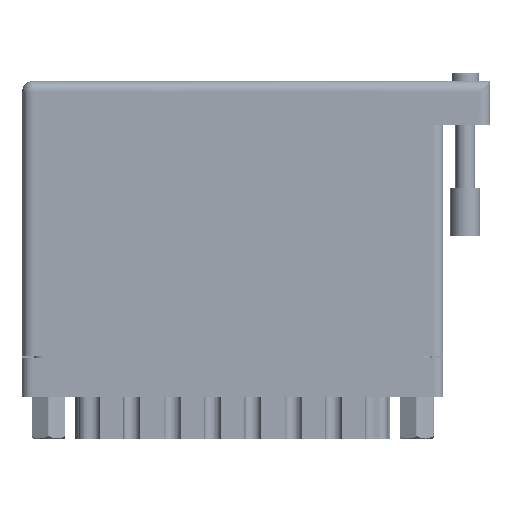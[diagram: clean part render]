
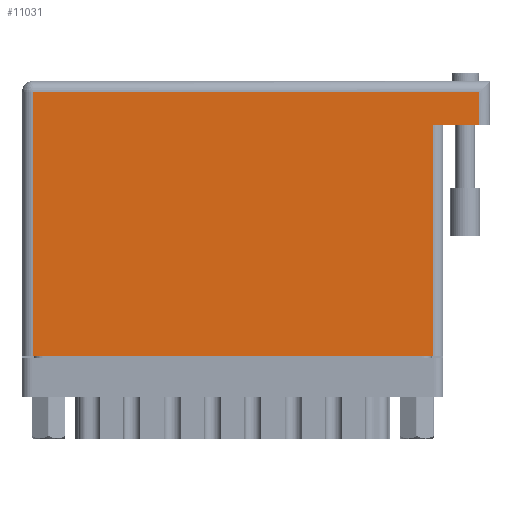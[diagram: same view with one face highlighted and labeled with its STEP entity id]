
A CAD part, front view. The second image highlights one B-rep face of the part: STEP entity #11031.
In plain terms, the highlighted face is planar.
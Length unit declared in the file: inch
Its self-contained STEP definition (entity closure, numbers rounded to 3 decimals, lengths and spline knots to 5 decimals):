
#3420 = ORIENTED_EDGE ( 'NONE', *, *, #61416, .T. ) ;
#5958 = DIRECTION ( 'NONE',  ( 1., 0., 0. ) ) ;
#5983 = AXIS2_PLACEMENT_3D ( 'NONE', #17333, #24297, #83875 ) ;
#5984 = EDGE_CURVE ( 'NONE', #15269, #26244, #51164, .T. ) ;
#6427 = CARTESIAN_POINT ( 'NONE',  ( 0.07, 0., 0. ) ) ;
#7110 = DIRECTION ( 'NONE',  ( 0., 1., 0. ) ) ;
#8428 = ORIENTED_EDGE ( 'NONE', *, *, #5984, .T. ) ;
#8669 = FACE_OUTER_BOUND ( 'NONE', #66862, .T. ) ;
#9192 = LINE ( 'NONE', #63873, #42277 ) ;
#9194 = LINE ( 'NONE', #27393, #59892 ) ;
#9333 = EDGE_CURVE ( 'NONE', #26244, #36953, #9194, .T. ) ;
#11031 = ADVANCED_FACE ( 'NONE', ( #8669 ), #83304, .F. ) ;
#11588 = VERTEX_POINT ( 'NONE', #49985 ) ;
#12698 = LINE ( 'NONE', #33693, #57027 ) ;
#13723 = DIRECTION ( 'NONE',  ( -1., 0., 0. ) ) ;
#15269 = VERTEX_POINT ( 'NONE', #6427 ) ;
#17333 = CARTESIAN_POINT ( 'NONE',  ( 0., 1.775, 0. ) ) ;
#22354 = ORIENTED_EDGE ( 'NONE', *, *, #35326, .T. ) ;
#23935 = EDGE_CURVE ( 'NONE', #74071, #11588, #73163, .T. ) ;
#24273 = DIRECTION ( 'NONE',  ( 0., -1., 0. ) ) ;
#24297 = DIRECTION ( 'NONE',  ( 0., 0., -1. ) ) ;
#25560 = EDGE_CURVE ( 'NONE', #74071, #36953, #12698, .T. ) ;
#26244 = VERTEX_POINT ( 'NONE', #29284 ) ;
#27393 = CARTESIAN_POINT ( 'NONE',  ( 2.648, 1.495, 0. ) ) ;
#29284 = CARTESIAN_POINT ( 'NONE',  ( 2.648, 0., 0. ) ) ;
#32236 = ORIENTED_EDGE ( 'NONE', *, *, #25560, .F. ) ;
#33693 = CARTESIAN_POINT ( 'NONE',  ( 3.018, 1.495, 0. ) ) ;
#35326 = EDGE_CURVE ( 'NONE', #11588, #36630, #79288, .T. ) ;
#36630 = VERTEX_POINT ( 'NONE', #47289 ) ;
#36953 = VERTEX_POINT ( 'NONE', #84575 ) ;
#42277 = VECTOR ( 'NONE', #24273, 39.37008 ) ;
#47289 = CARTESIAN_POINT ( 'NONE',  ( 0.07, 1.705, 0. ) ) ;
#49985 = CARTESIAN_POINT ( 'NONE',  ( 2.948, 1.705, 0. ) ) ;
#51164 = LINE ( 'NONE', #84972, #66567 ) ;
#52670 = ORIENTED_EDGE ( 'NONE', *, *, #9333, .T. ) ;
#54772 = DIRECTION ( 'NONE',  ( 0., 1., 0. ) ) ;
#57027 = VECTOR ( 'NONE', #13723, 39.37008 ) ;
#59271 = ORIENTED_EDGE ( 'NONE', *, *, #23935, .T. ) ;
#59892 = VECTOR ( 'NONE', #7110, 39.37008 ) ;
#60761 = DIRECTION ( 'NONE',  ( -1., 0., 0. ) ) ;
#61416 = EDGE_CURVE ( 'NONE', #36630, #15269, #9192, .T. ) ;
#63873 = CARTESIAN_POINT ( 'NONE',  ( 0.07, 0., 0. ) ) ;
#65861 = VECTOR ( 'NONE', #60761, 39.37008 ) ;
#66567 = VECTOR ( 'NONE', #5958, 39.37008 ) ;
#66862 = EDGE_LOOP ( 'NONE', ( #8428, #52670, #32236, #59271, #22354, #3420 ) ) ;
#68002 = CARTESIAN_POINT ( 'NONE',  ( 2.948, 1.775, 0. ) ) ;
#68988 = VECTOR ( 'NONE', #54772, 39.37008 ) ;
#72067 = CARTESIAN_POINT ( 'NONE',  ( 2.948, 1.495, 0. ) ) ;
#73163 = LINE ( 'NONE', #68002, #68988 ) ;
#74039 = CARTESIAN_POINT ( 'NONE',  ( 0., 1.705, 0. ) ) ;
#74071 = VERTEX_POINT ( 'NONE', #72067 ) ;
#79288 = LINE ( 'NONE', #74039, #65861 ) ;
#83304 = PLANE ( 'NONE',  #5983 ) ;
#83875 = DIRECTION ( 'NONE',  ( -1., 0., 0. ) ) ;
#84575 = CARTESIAN_POINT ( 'NONE',  ( 2.648, 1.495, 0. ) ) ;
#84972 = CARTESIAN_POINT ( 'NONE',  ( 0., 0., 0. ) ) ;
